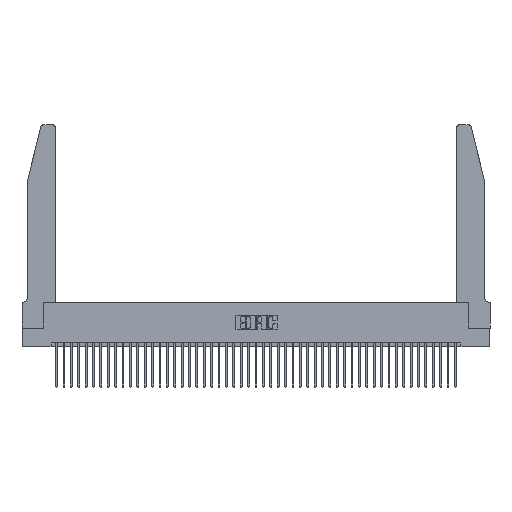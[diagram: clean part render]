
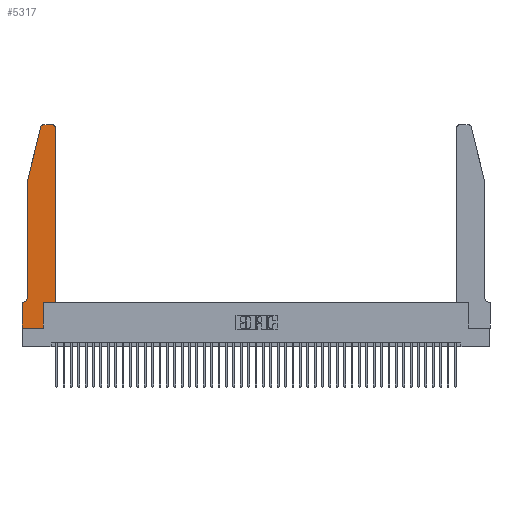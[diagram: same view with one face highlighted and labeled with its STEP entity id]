
A CAD part, top view. The second image highlights one B-rep face of the part: STEP entity #5317.
In plain terms, the highlighted planar face has unit normal (0, 0, 1).
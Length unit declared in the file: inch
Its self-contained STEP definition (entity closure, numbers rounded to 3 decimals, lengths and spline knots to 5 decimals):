
#144 = LINE ( 'NONE', #1943, #9730 ) ;
#969 = CARTESIAN_POINT ( 'NONE',  ( 0.0055, 0.42, 0.37 ) ) ;
#1026 = DIRECTION ( 'NONE',  ( 0., 1., 0. ) ) ;
#1191 = EDGE_CURVE ( 'NONE', #9293, #39585, #144, .T. ) ;
#1406 = LINE ( 'NONE', #25920, #44371 ) ;
#1943 = CARTESIAN_POINT ( 'NONE',  ( 0., 0., 0.37 ) ) ;
#2385 = VERTEX_POINT ( 'NONE', #36400 ) ;
#2480 = DIRECTION ( 'NONE',  ( 0., 1., 0. ) ) ;
#3142 = EDGE_CURVE ( 'NONE', #2385, #43464, #18639, .T. ) ;
#3185 = CARTESIAN_POINT ( 'NONE',  ( 0.0755, 2., 0.37 ) ) ;
#3530 = EDGE_CURVE ( 'NONE', #31772, #2385, #36395, .T. ) ;
#3968 = CARTESIAN_POINT ( 'NONE',  ( 0.0755, 2., 0.37 ) ) ;
#4331 = CARTESIAN_POINT ( 'NONE',  ( 0.4505, 2.72, 0.37 ) ) ;
#4563 = DIRECTION ( 'NONE',  ( -1., 0., 0. ) ) ;
#4630 = DIRECTION ( 'NONE',  ( 0., 0., 1. ) ) ;
#5317 = ADVANCED_FACE ( 'NONE', ( #39520 ), #26126, .T. ) ;
#5382 = DIRECTION ( 'NONE',  ( -1., 0., 0. ) ) ;
#5449 = EDGE_LOOP ( 'NONE', ( #33711, #20959, #45852, #24817, #29784, #45277, #24261, #41932, #23154, #20922, #38656, #17528 ) ) ;
#5978 = VERTEX_POINT ( 'NONE', #7948 ) ;
#7213 = EDGE_CURVE ( 'NONE', #21139, #28720, #30201, .T. ) ;
#7682 = LINE ( 'NONE', #16272, #25668 ) ;
#7948 = CARTESIAN_POINT ( 'NONE',  ( 0.0055, 0.35, 0.37 ) ) ;
#8029 = LINE ( 'NONE', #40358, #28207 ) ;
#8562 = CARTESIAN_POINT ( 'NONE',  ( 0.284, 2.75, 0.37 ) ) ;
#8649 = DIRECTION ( 'NONE',  ( -1., 0., 0. ) ) ;
#8718 = CIRCLE ( 'NONE', #20366, 0.07 ) ;
#9293 = VERTEX_POINT ( 'NONE', #22401 ) ;
#9730 = VECTOR ( 'NONE', #16275, 39.37008 ) ;
#11681 = DIRECTION ( 'NONE',  ( 0., -1., 0. ) ) ;
#11990 = AXIS2_PLACEMENT_3D ( 'NONE', #16589, #41416, #20255 ) ;
#12052 = DIRECTION ( 'NONE',  ( 1., 0., 0. ) ) ;
#12656 = DIRECTION ( 'NONE',  ( 1., 0., 0. ) ) ;
#13105 = AXIS2_PLACEMENT_3D ( 'NONE', #36681, #4630, #29685 ) ;
#14863 = DIRECTION ( 'NONE',  ( -0.239, -0.971, 0. ) ) ;
#16272 = CARTESIAN_POINT ( 'NONE',  ( 0.0755, 0.35, 0.37 ) ) ;
#16275 = DIRECTION ( 'NONE',  ( 0., -1., 0. ) ) ;
#16589 = CARTESIAN_POINT ( 'NONE',  ( 0.284, 2.72, 0.37 ) ) ;
#17528 = ORIENTED_EDGE ( 'NONE', *, *, #22800, .T. ) ;
#18639 = LINE ( 'NONE', #20457, #23688 ) ;
#18936 = AXIS2_PLACEMENT_3D ( 'NONE', #41507, #20339, #45070 ) ;
#19332 = VECTOR ( 'NONE', #12656, 39.37008 ) ;
#20255 = DIRECTION ( 'NONE',  ( 1., 0., 0. ) ) ;
#20339 = DIRECTION ( 'NONE',  ( 0., 0., 1. ) ) ;
#20366 = AXIS2_PLACEMENT_3D ( 'NONE', #969, #26065, #4563 ) ;
#20457 = CARTESIAN_POINT ( 'NONE',  ( 0.4505, 0.35, 0.37 ) ) ;
#20922 = ORIENTED_EDGE ( 'NONE', *, *, #3530, .T. ) ;
#20959 = ORIENTED_EDGE ( 'NONE', *, *, #33306, .T. ) ;
#21139 = VERTEX_POINT ( 'NONE', #31599 ) ;
#22053 = CARTESIAN_POINT ( 'NONE',  ( 0., 0., 0.37 ) ) ;
#22169 = EDGE_CURVE ( 'NONE', #39585, #38896, #28739, .T. ) ;
#22401 = CARTESIAN_POINT ( 'NONE',  ( 0., 0.35, 0.37 ) ) ;
#22800 = EDGE_CURVE ( 'NONE', #43464, #21139, #41968, .T. ) ;
#22939 = CIRCLE ( 'NONE', #11990, 0.03 ) ;
#23154 = ORIENTED_EDGE ( 'NONE', *, *, #30406, .T. ) ;
#23688 = VECTOR ( 'NONE', #2480, 39.37008 ) ;
#24261 = ORIENTED_EDGE ( 'NONE', *, *, #1191, .T. ) ;
#24817 = ORIENTED_EDGE ( 'NONE', *, *, #29226, .T. ) ;
#25668 = VECTOR ( 'NONE', #5382, 39.37008 ) ;
#25920 = CARTESIAN_POINT ( 'NONE',  ( 0.0755, 2., 0.37 ) ) ;
#26065 = DIRECTION ( 'NONE',  ( 0., 0., -1. ) ) ;
#26126 = PLANE ( 'NONE',  #13105 ) ;
#26943 = VECTOR ( 'NONE', #12052, 39.37008 ) ;
#27654 = CARTESIAN_POINT ( 'NONE',  ( 0.0755, 0.42, 0.37 ) ) ;
#27954 = VECTOR ( 'NONE', #8649, 39.37008 ) ;
#28207 = VECTOR ( 'NONE', #1026, 39.37008 ) ;
#28415 = CARTESIAN_POINT ( 'NONE',  ( 0.25487, 2.72718, 0.37 ) ) ;
#28720 = VERTEX_POINT ( 'NONE', #8562 ) ;
#28739 = LINE ( 'NONE', #40934, #19332 ) ;
#29161 = LINE ( 'NONE', #3968, #45765 ) ;
#29226 = EDGE_CURVE ( 'NONE', #35383, #35284, #1406, .T. ) ;
#29231 = EDGE_CURVE ( 'NONE', #35284, #5978, #8718, .T. ) ;
#29685 = DIRECTION ( 'NONE',  ( 1., 0., 0. ) ) ;
#29784 = ORIENTED_EDGE ( 'NONE', *, *, #29231, .T. ) ;
#29837 = CARTESIAN_POINT ( 'NONE',  ( 0.4505, 0.35, 0.37 ) ) ;
#30201 = LINE ( 'NONE', #44143, #27954 ) ;
#30406 = EDGE_CURVE ( 'NONE', #38896, #31772, #8029, .T. ) ;
#30833 = CARTESIAN_POINT ( 'NONE',  ( 0.2865, 0.35, 0.37 ) ) ;
#30837 = VERTEX_POINT ( 'NONE', #28415 ) ;
#31599 = CARTESIAN_POINT ( 'NONE',  ( 0.4205, 2.75, 0.37 ) ) ;
#31772 = VERTEX_POINT ( 'NONE', #30833 ) ;
#33306 = EDGE_CURVE ( 'NONE', #28720, #30837, #22939, .T. ) ;
#33711 = ORIENTED_EDGE ( 'NONE', *, *, #7213, .T. ) ;
#35164 = CARTESIAN_POINT ( 'NONE',  ( 0.2865, 0., 0.37 ) ) ;
#35284 = VERTEX_POINT ( 'NONE', #27654 ) ;
#35383 = VERTEX_POINT ( 'NONE', #3185 ) ;
#36395 = LINE ( 'NONE', #29837, #26943 ) ;
#36400 = CARTESIAN_POINT ( 'NONE',  ( 0.4505, 0.35, 0.37 ) ) ;
#36681 = CARTESIAN_POINT ( 'NONE',  ( 0., 0.35, 0.37 ) ) ;
#38656 = ORIENTED_EDGE ( 'NONE', *, *, #3142, .T. ) ;
#38896 = VERTEX_POINT ( 'NONE', #35164 ) ;
#39520 = FACE_OUTER_BOUND ( 'NONE', #5449, .T. ) ;
#39585 = VERTEX_POINT ( 'NONE', #22053 ) ;
#40358 = CARTESIAN_POINT ( 'NONE',  ( 0.2865, 0.35, 0.37 ) ) ;
#40934 = CARTESIAN_POINT ( 'NONE',  ( 0., 0., 0.37 ) ) ;
#41416 = DIRECTION ( 'NONE',  ( 0., 0., 1. ) ) ;
#41507 = CARTESIAN_POINT ( 'NONE',  ( 0.4205, 2.72, 0.37 ) ) ;
#41932 = ORIENTED_EDGE ( 'NONE', *, *, #22169, .T. ) ;
#41968 = CIRCLE ( 'NONE', #18936, 0.03 ) ;
#42404 = EDGE_CURVE ( 'NONE', #5978, #9293, #7682, .T. ) ;
#43464 = VERTEX_POINT ( 'NONE', #4331 ) ;
#44143 = CARTESIAN_POINT ( 'NONE',  ( 0.2605, 2.75, 0.37 ) ) ;
#44327 = EDGE_CURVE ( 'NONE', #30837, #35383, #29161, .T. ) ;
#44371 = VECTOR ( 'NONE', #11681, 39.37008 ) ;
#45070 = DIRECTION ( 'NONE',  ( 1., 0., 0. ) ) ;
#45277 = ORIENTED_EDGE ( 'NONE', *, *, #42404, .T. ) ;
#45765 = VECTOR ( 'NONE', #14863, 39.37008 ) ;
#45852 = ORIENTED_EDGE ( 'NONE', *, *, #44327, .T. ) ;
